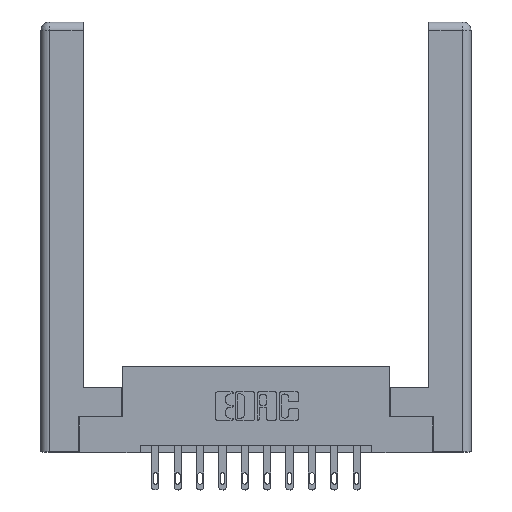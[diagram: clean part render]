
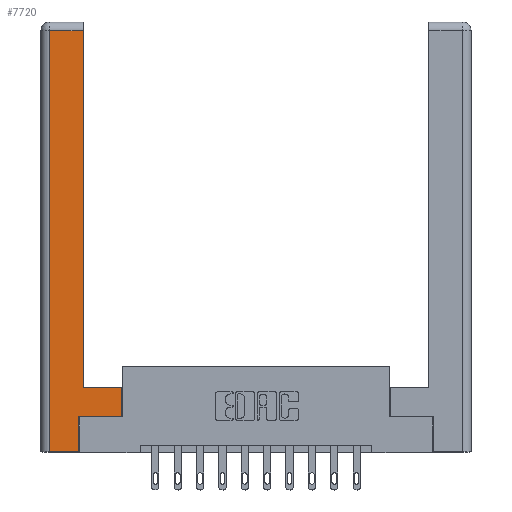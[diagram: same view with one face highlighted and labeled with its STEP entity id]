
A CAD part, top view. The second image highlights one B-rep face of the part: STEP entity #7720.
In plain terms, the highlighted planar face has unit normal (0, 0, 1).
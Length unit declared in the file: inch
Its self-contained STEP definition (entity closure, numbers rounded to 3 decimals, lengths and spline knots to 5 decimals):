
#439 = FACE_OUTER_BOUND ( 'NONE', #3479, .T. ) ;
#1013 = LINE ( 'NONE', #6681, #4864 ) ;
#1289 = VERTEX_POINT ( 'NONE', #10956 ) ;
#1654 = VECTOR ( 'NONE', #6435, 39.37008 ) ;
#1807 = VERTEX_POINT ( 'NONE', #3983 ) ;
#1925 = ORIENTED_EDGE ( 'NONE', *, *, #11105, .T. ) ;
#2527 = EDGE_CURVE ( 'NONE', #10353, #7229, #9833, .T. ) ;
#2594 = VERTEX_POINT ( 'NONE', #11385 ) ;
#2873 = CARTESIAN_POINT ( 'NONE',  ( 0.295, 2.94, 0. ) ) ;
#2953 = DIRECTION ( 'NONE',  ( -1., 0., 0. ) ) ;
#3479 = EDGE_LOOP ( 'NONE', ( #4652, #13859, #4843, #5760, #12220, #9363, #1925, #8826 ) ) ;
#3983 = CARTESIAN_POINT ( 'NONE',  ( 0.265, 0.245, 0. ) ) ;
#4079 = CARTESIAN_POINT ( 'NONE',  ( 0.0615, 2.94, 0. ) ) ;
#4132 = AXIS2_PLACEMENT_3D ( 'NONE', #14152, #7469, #2953 ) ;
#4445 = CARTESIAN_POINT ( 'NONE',  ( 0.0615, 0., 0. ) ) ;
#4493 = CARTESIAN_POINT ( 'NONE',  ( 0.565, 0.245, 0. ) ) ;
#4632 = DIRECTION ( 'NONE',  ( 1., 0., 0. ) ) ;
#4652 = ORIENTED_EDGE ( 'NONE', *, *, #2527, .T. ) ;
#4738 = CARTESIAN_POINT ( 'NONE',  ( 0.295, 0.45, 0. ) ) ;
#4742 = VECTOR ( 'NONE', #5212, 39.37008 ) ;
#4801 = LINE ( 'NONE', #6362, #5844 ) ;
#4843 = ORIENTED_EDGE ( 'NONE', *, *, #6703, .T. ) ;
#4864 = VECTOR ( 'NONE', #7912, 39.37008 ) ;
#4984 = LINE ( 'NONE', #6343, #1654 ) ;
#5212 = DIRECTION ( 'NONE',  ( -1., 0., 0. ) ) ;
#5718 = CARTESIAN_POINT ( 'NONE',  ( 0.295, 3., 0. ) ) ;
#5760 = ORIENTED_EDGE ( 'NONE', *, *, #12138, .T. ) ;
#5844 = VECTOR ( 'NONE', #13067, 39.37008 ) ;
#6343 = CARTESIAN_POINT ( 'NONE',  ( 0.0615, 0., 0. ) ) ;
#6362 = CARTESIAN_POINT ( 'NONE',  ( 0.265, 0.245, 0. ) ) ;
#6435 = DIRECTION ( 'NONE',  ( 0., -1., 0. ) ) ;
#6681 = CARTESIAN_POINT ( 'NONE',  ( 0.265, 0., 0. ) ) ;
#6685 = EDGE_CURVE ( 'NONE', #1289, #10353, #7085, .T. ) ;
#6703 = EDGE_CURVE ( 'NONE', #10693, #13243, #4984, .T. ) ;
#6902 = VECTOR ( 'NONE', #12056, 39.37008 ) ;
#7085 = LINE ( 'NONE', #7689, #6902 ) ;
#7229 = VERTEX_POINT ( 'NONE', #2873 ) ;
#7352 = VECTOR ( 'NONE', #13954, 39.37008 ) ;
#7469 = DIRECTION ( 'NONE',  ( 0., 0., -1. ) ) ;
#7689 = CARTESIAN_POINT ( 'NONE',  ( 0.295, 0.45, 0. ) ) ;
#7720 = ADVANCED_FACE ( 'NONE', ( #439 ), #12976, .F. ) ;
#7912 = DIRECTION ( 'NONE',  ( 1., 0., 0. ) ) ;
#7969 = EDGE_CURVE ( 'NONE', #10512, #1807, #4801, .T. ) ;
#8249 = LINE ( 'NONE', #4493, #9110 ) ;
#8826 = ORIENTED_EDGE ( 'NONE', *, *, #6685, .T. ) ;
#9110 = VECTOR ( 'NONE', #4632, 39.37008 ) ;
#9363 = ORIENTED_EDGE ( 'NONE', *, *, #10179, .T. ) ;
#9431 = LINE ( 'NONE', #10375, #7352 ) ;
#9623 = LINE ( 'NONE', #4079, #4742 ) ;
#9833 = LINE ( 'NONE', #5718, #13167 ) ;
#10179 = EDGE_CURVE ( 'NONE', #1807, #2594, #8249, .T. ) ;
#10213 = DIRECTION ( 'NONE',  ( 0., 1., 0. ) ) ;
#10353 = VERTEX_POINT ( 'NONE', #4738 ) ;
#10375 = CARTESIAN_POINT ( 'NONE',  ( 0.565, 0.45, 0. ) ) ;
#10512 = VERTEX_POINT ( 'NONE', #12884 ) ;
#10584 = EDGE_CURVE ( 'NONE', #7229, #10693, #9623, .T. ) ;
#10693 = VERTEX_POINT ( 'NONE', #12139 ) ;
#10956 = CARTESIAN_POINT ( 'NONE',  ( 0.565, 0.45, 0. ) ) ;
#11105 = EDGE_CURVE ( 'NONE', #2594, #1289, #9431, .T. ) ;
#11385 = CARTESIAN_POINT ( 'NONE',  ( 0.565, 0.245, 0. ) ) ;
#12056 = DIRECTION ( 'NONE',  ( -1., 0., 0. ) ) ;
#12138 = EDGE_CURVE ( 'NONE', #13243, #10512, #1013, .T. ) ;
#12139 = CARTESIAN_POINT ( 'NONE',  ( 0.0615, 2.94, 0. ) ) ;
#12220 = ORIENTED_EDGE ( 'NONE', *, *, #7969, .T. ) ;
#12884 = CARTESIAN_POINT ( 'NONE',  ( 0.265, 0., 0. ) ) ;
#12976 = PLANE ( 'NONE',  #4132 ) ;
#13067 = DIRECTION ( 'NONE',  ( 0., 1., 0. ) ) ;
#13167 = VECTOR ( 'NONE', #10213, 39.37008 ) ;
#13243 = VERTEX_POINT ( 'NONE', #4445 ) ;
#13859 = ORIENTED_EDGE ( 'NONE', *, *, #10584, .T. ) ;
#13954 = DIRECTION ( 'NONE',  ( 0., 1., 0. ) ) ;
#14152 = CARTESIAN_POINT ( 'NONE',  ( 0., 0., 0. ) ) ;
